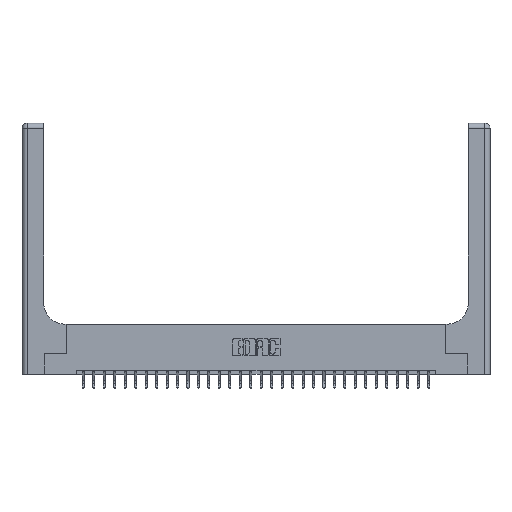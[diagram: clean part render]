
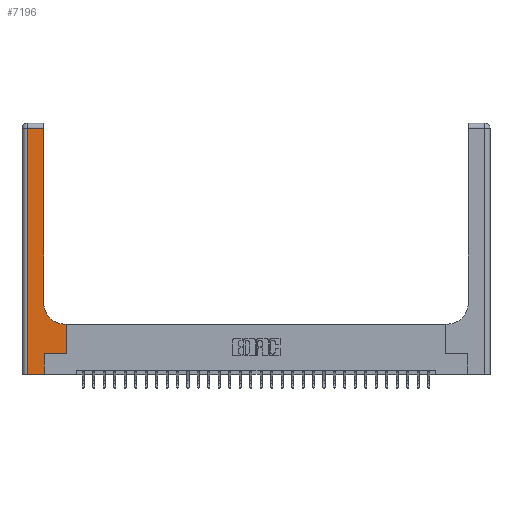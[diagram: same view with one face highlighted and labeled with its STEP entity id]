
A CAD part, top view. The second image highlights one B-rep face of the part: STEP entity #7196.
In plain terms, the highlighted planar face has unit normal (0, 0, 1).
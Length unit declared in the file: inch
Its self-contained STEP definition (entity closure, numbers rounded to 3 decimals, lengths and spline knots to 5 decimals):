
#466 = CARTESIAN_POINT ( 'NONE',  ( 0.26, 0.6, 0.37 ) ) ;
#758 = DIRECTION ( 'NONE',  ( -1., 0., 0. ) ) ;
#1207 = PLANE ( 'NONE',  #10174 ) ;
#1261 = CARTESIAN_POINT ( 'NONE',  ( 0.06, 2.94, 0.37 ) ) ;
#1349 = LINE ( 'NONE', #12528, #26240 ) ;
#1547 = CARTESIAN_POINT ( 'NONE',  ( 0.265, 0., 0.37 ) ) ;
#1787 = LINE ( 'NONE', #18139, #16890 ) ;
#1850 = CARTESIAN_POINT ( 'NONE',  ( 0.06, 3., 0.37 ) ) ;
#1972 = CIRCLE ( 'NONE', #4840, 0.25 ) ;
#2183 = ORIENTED_EDGE ( 'NONE', *, *, #4704, .T. ) ;
#2483 = DIRECTION ( 'NONE',  ( -1., 0., 0. ) ) ;
#2587 = ORIENTED_EDGE ( 'NONE', *, *, #23220, .T. ) ;
#3761 = LINE ( 'NONE', #1547, #19975 ) ;
#3892 = CARTESIAN_POINT ( 'NONE',  ( 0.51, 0.6, 0.37 ) ) ;
#4483 = CARTESIAN_POINT ( 'NONE',  ( 0.528, 0.25, 0.37 ) ) ;
#4704 = EDGE_CURVE ( 'NONE', #27287, #6442, #19712, .T. ) ;
#4840 = AXIS2_PLACEMENT_3D ( 'NONE', #20393, #15534, #26890 ) ;
#4987 = DIRECTION ( 'NONE',  ( 0., 0., -1. ) ) ;
#5069 = VECTOR ( 'NONE', #10675, 39.37008 ) ;
#5101 = VERTEX_POINT ( 'NONE', #3892 ) ;
#5745 = VERTEX_POINT ( 'NONE', #23443 ) ;
#5871 = CARTESIAN_POINT ( 'NONE',  ( 0.265, 0.25, 0.37 ) ) ;
#6256 = EDGE_CURVE ( 'NONE', #27533, #5745, #13319, .T. ) ;
#6442 = VERTEX_POINT ( 'NONE', #24836 ) ;
#7196 = ADVANCED_FACE ( 'NONE', ( #22529 ), #1207, .F. ) ;
#8246 = DIRECTION ( 'NONE',  ( 1., 0., 0. ) ) ;
#8669 = ORIENTED_EDGE ( 'NONE', *, *, #20234, .T. ) ;
#8802 = VERTEX_POINT ( 'NONE', #21864 ) ;
#8828 = DIRECTION ( 'NONE',  ( -1., 0., 0. ) ) ;
#9375 = ORIENTED_EDGE ( 'NONE', *, *, #14891, .T. ) ;
#9480 = CARTESIAN_POINT ( 'NONE',  ( 0.26, 0.85, 0.37 ) ) ;
#10029 = EDGE_CURVE ( 'NONE', #16712, #8802, #3761, .T. ) ;
#10174 = AXIS2_PLACEMENT_3D ( 'NONE', #27121, #4987, #2483 ) ;
#10397 = ORIENTED_EDGE ( 'NONE', *, *, #10029, .T. ) ;
#10675 = DIRECTION ( 'NONE',  ( 0., -1., 0. ) ) ;
#10738 = CARTESIAN_POINT ( 'NONE',  ( 0.265, 0., 0.37 ) ) ;
#11122 = VERTEX_POINT ( 'NONE', #27118 ) ;
#12528 = CARTESIAN_POINT ( 'NONE',  ( 0., 0., 0.37 ) ) ;
#12882 = EDGE_CURVE ( 'NONE', #14984, #11122, #18117, .T. ) ;
#13319 = LINE ( 'NONE', #1850, #5069 ) ;
#13499 = DIRECTION ( 'NONE',  ( 0., 1., 0. ) ) ;
#13671 = ORIENTED_EDGE ( 'NONE', *, *, #23086, .T. ) ;
#13967 = CARTESIAN_POINT ( 'NONE',  ( 0.528, 0.25, 0.37 ) ) ;
#14815 = DIRECTION ( 'NONE',  ( 0., 1., 0. ) ) ;
#14891 = EDGE_CURVE ( 'NONE', #5101, #27287, #1972, .T. ) ;
#14984 = VERTEX_POINT ( 'NONE', #4483 ) ;
#15159 = LINE ( 'NONE', #5871, #27143 ) ;
#15305 = DIRECTION ( 'NONE',  ( 1., 0., 0. ) ) ;
#15534 = DIRECTION ( 'NONE',  ( 0., 0., -1. ) ) ;
#15539 = ORIENTED_EDGE ( 'NONE', *, *, #6256, .T. ) ;
#16712 = VERTEX_POINT ( 'NONE', #10738 ) ;
#16890 = VECTOR ( 'NONE', #8828, 39.37008 ) ;
#18010 = VECTOR ( 'NONE', #24897, 39.37008 ) ;
#18117 = LINE ( 'NONE', #13967, #18010 ) ;
#18139 = CARTESIAN_POINT ( 'NONE',  ( 0., 2.94, 0.37 ) ) ;
#19712 = LINE ( 'NONE', #22046, #24481 ) ;
#19975 = VECTOR ( 'NONE', #14815, 39.37008 ) ;
#20234 = EDGE_CURVE ( 'NONE', #8802, #14984, #15159, .T. ) ;
#20393 = CARTESIAN_POINT ( 'NONE',  ( 0.51, 0.85, 0.37 ) ) ;
#20550 = EDGE_LOOP ( 'NONE', ( #2183, #27241, #15539, #2587, #10397, #8669, #28999, #13671, #9375 ) ) ;
#20654 = LINE ( 'NONE', #466, #22449 ) ;
#21864 = CARTESIAN_POINT ( 'NONE',  ( 0.265, 0.25, 0.37 ) ) ;
#22046 = CARTESIAN_POINT ( 'NONE',  ( 0.26, 3., 0.37 ) ) ;
#22449 = VECTOR ( 'NONE', #758, 39.37008 ) ;
#22529 = FACE_OUTER_BOUND ( 'NONE', #20550, .T. ) ;
#23086 = EDGE_CURVE ( 'NONE', #11122, #5101, #20654, .T. ) ;
#23220 = EDGE_CURVE ( 'NONE', #5745, #16712, #1349, .T. ) ;
#23443 = CARTESIAN_POINT ( 'NONE',  ( 0.06, 0., 0.37 ) ) ;
#24481 = VECTOR ( 'NONE', #13499, 39.37008 ) ;
#24836 = CARTESIAN_POINT ( 'NONE',  ( 0.26, 2.94, 0.37 ) ) ;
#24897 = DIRECTION ( 'NONE',  ( 0., 1., 0. ) ) ;
#25021 = EDGE_CURVE ( 'NONE', #6442, #27533, #1787, .T. ) ;
#26240 = VECTOR ( 'NONE', #8246, 39.37008 ) ;
#26890 = DIRECTION ( 'NONE',  ( 1., 0., 0. ) ) ;
#27118 = CARTESIAN_POINT ( 'NONE',  ( 0.528, 0.6, 0.37 ) ) ;
#27121 = CARTESIAN_POINT ( 'NONE',  ( 0., 3., 0.37 ) ) ;
#27143 = VECTOR ( 'NONE', #15305, 39.37008 ) ;
#27241 = ORIENTED_EDGE ( 'NONE', *, *, #25021, .T. ) ;
#27287 = VERTEX_POINT ( 'NONE', #9480 ) ;
#27533 = VERTEX_POINT ( 'NONE', #1261 ) ;
#28999 = ORIENTED_EDGE ( 'NONE', *, *, #12882, .T. ) ;
